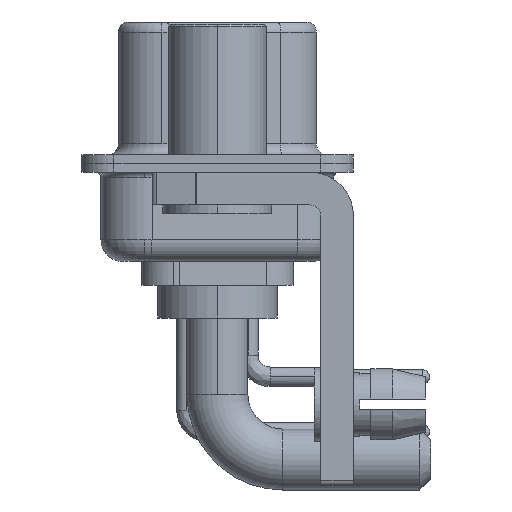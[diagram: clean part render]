
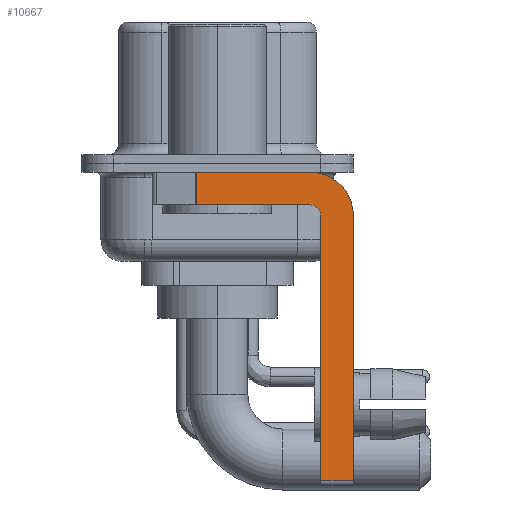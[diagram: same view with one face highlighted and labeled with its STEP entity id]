
A CAD part, left-side view. The second image highlights one B-rep face of the part: STEP entity #10667.
In plain terms, the highlighted planar face has unit normal (-1, 0, 0).
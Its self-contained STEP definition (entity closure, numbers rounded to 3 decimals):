
#147 = VERTEX_POINT ( 'NONE', #17949 ) ;
#421 = CIRCLE ( 'NONE', #19704, 0.5 ) ;
#507 = EDGE_CURVE ( 'NONE', #19355, #1604, #15994, .T. ) ;
#1159 = CIRCLE ( 'NONE', #16496, 2. ) ;
#1604 = VERTEX_POINT ( 'NONE', #11818 ) ;
#2180 = ORIENTED_EDGE ( 'NONE', *, *, #14602, .T. ) ;
#2660 = DIRECTION ( 'NONE',  ( 0., 0., 1. ) ) ;
#2779 = LINE ( 'NONE', #15398, #18333 ) ;
#2852 = DIRECTION ( 'NONE',  ( -1., 0., 0. ) ) ;
#2991 = CARTESIAN_POINT ( 'NONE',  ( -2.9, -6.25, -14.55 ) ) ;
#3131 = ORIENTED_EDGE ( 'NONE', *, *, #14201, .F. ) ;
#3247 = DIRECTION ( 'NONE',  ( 0., -1., 0. ) ) ;
#4165 = VECTOR ( 'NONE', #14245, 1000. ) ;
#4383 = VERTEX_POINT ( 'NONE', #23529 ) ;
#4428 = CARTESIAN_POINT ( 'NONE',  ( -2.9, 0.978, -1.9 ) ) ;
#4483 = CARTESIAN_POINT ( 'NONE',  ( -2.9, 0.978, -1.9 ) ) ;
#5187 = VERTEX_POINT ( 'NONE', #22935 ) ;
#5738 = DIRECTION ( 'NONE',  ( 0., 0., -1. ) ) ;
#6013 = ORIENTED_EDGE ( 'NONE', *, *, #7132, .F. ) ;
#6965 = EDGE_CURVE ( 'NONE', #1604, #4383, #1159, .T. ) ;
#7058 = CARTESIAN_POINT ( 'NONE',  ( -2.9, -4.75, -14.8 ) ) ;
#7132 = EDGE_CURVE ( 'NONE', #147, #17319, #421, .T. ) ;
#7794 = FACE_OUTER_BOUND ( 'NONE', #13301, .T. ) ;
#7933 = CARTESIAN_POINT ( 'NONE',  ( -2.9, -4.25, -2.4 ) ) ;
#8340 = LINE ( 'NONE', #7058, #17903 ) ;
#8738 = VECTOR ( 'NONE', #19091, 1000. ) ;
#9876 = CARTESIAN_POINT ( 'NONE',  ( -2.9, -6.25, -2.4 ) ) ;
#10667 = ADVANCED_FACE ( 'NONE', ( #7794 ), #14624, .F. ) ;
#10723 = LINE ( 'NONE', #4428, #8738 ) ;
#10788 = VERTEX_POINT ( 'NONE', #4483 ) ;
#11657 = CARTESIAN_POINT ( 'NONE',  ( -2.9, 0.978, -0.4 ) ) ;
#11818 = CARTESIAN_POINT ( 'NONE',  ( -2.9, -4.25, -0.4 ) ) ;
#12243 = VECTOR ( 'NONE', #3247, 1000. ) ;
#12498 = ORIENTED_EDGE ( 'NONE', *, *, #21752, .F. ) ;
#12738 = EDGE_CURVE ( 'NONE', #5187, #26449, #2779, .T. ) ;
#13301 = EDGE_LOOP ( 'NONE', ( #15596, #2180, #12498, #6013, #3131, #19892, #27076, #26607 ) ) ;
#14146 = CARTESIAN_POINT ( 'NONE',  ( -2.9, -4.25, -1.9 ) ) ;
#14201 = EDGE_CURVE ( 'NONE', #5187, #147, #8340, .T. ) ;
#14245 = DIRECTION ( 'NONE',  ( 0., 0., -1. ) ) ;
#14602 = EDGE_CURVE ( 'NONE', #19355, #10788, #10723, .T. ) ;
#14624 = PLANE ( 'NONE',  #25713 ) ;
#15398 = CARTESIAN_POINT ( 'NONE',  ( -2.9, -4.25, -14.55 ) ) ;
#15446 = CARTESIAN_POINT ( 'NONE',  ( -2.9, 3., -0.4 ) ) ;
#15596 = ORIENTED_EDGE ( 'NONE', *, *, #507, .F. ) ;
#15994 = LINE ( 'NONE', #15446, #12243 ) ;
#16496 = AXIS2_PLACEMENT_3D ( 'NONE', #18379, #25230, #26882 ) ;
#17062 = DIRECTION ( 'NONE',  ( 0., -1., 0. ) ) ;
#17319 = VERTEX_POINT ( 'NONE', #19640 ) ;
#17903 = VECTOR ( 'NONE', #2660, 1000. ) ;
#17949 = CARTESIAN_POINT ( 'NONE',  ( -2.9, -4.75, -2.4 ) ) ;
#18227 = LINE ( 'NONE', #9876, #4165 ) ;
#18333 = VECTOR ( 'NONE', #17062, 1000. ) ;
#18379 = CARTESIAN_POINT ( 'NONE',  ( -2.9, -4.25, -2.4 ) ) ;
#19091 = DIRECTION ( 'NONE',  ( 0., 0., -1. ) ) ;
#19322 = DIRECTION ( 'NONE',  ( 0., 0., 1. ) ) ;
#19355 = VERTEX_POINT ( 'NONE', #11657 ) ;
#19640 = CARTESIAN_POINT ( 'NONE',  ( -2.9, -4.25, -1.9 ) ) ;
#19704 = AXIS2_PLACEMENT_3D ( 'NONE', #25635, #2852, #19322 ) ;
#19892 = ORIENTED_EDGE ( 'NONE', *, *, #12738, .T. ) ;
#20336 = LINE ( 'NONE', #14146, #26478 ) ;
#20550 = DIRECTION ( 'NONE',  ( 1., 0., 0. ) ) ;
#21752 = EDGE_CURVE ( 'NONE', #17319, #10788, #20336, .T. ) ;
#22174 = EDGE_CURVE ( 'NONE', #4383, #26449, #18227, .T. ) ;
#22795 = DIRECTION ( 'NONE',  ( 0., 1., 0. ) ) ;
#22935 = CARTESIAN_POINT ( 'NONE',  ( -2.9, -4.75, -14.55 ) ) ;
#23529 = CARTESIAN_POINT ( 'NONE',  ( -2.9, -6.25, -2.4 ) ) ;
#25230 = DIRECTION ( 'NONE',  ( 1., 0., 0. ) ) ;
#25635 = CARTESIAN_POINT ( 'NONE',  ( -2.9, -4.25, -2.4 ) ) ;
#25713 = AXIS2_PLACEMENT_3D ( 'NONE', #7933, #20550, #5738 ) ;
#26449 = VERTEX_POINT ( 'NONE', #2991 ) ;
#26478 = VECTOR ( 'NONE', #22795, 1000. ) ;
#26607 = ORIENTED_EDGE ( 'NONE', *, *, #6965, .F. ) ;
#26882 = DIRECTION ( 'NONE',  ( 0., 0., -1. ) ) ;
#27076 = ORIENTED_EDGE ( 'NONE', *, *, #22174, .F. ) ;
